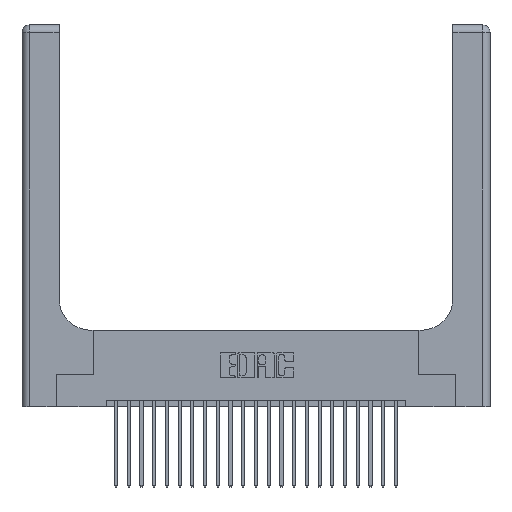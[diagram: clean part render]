
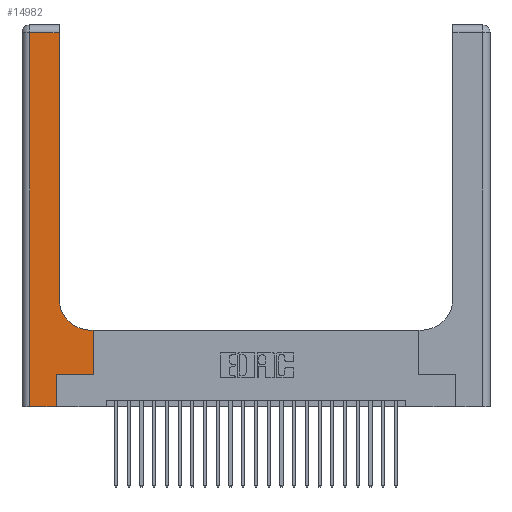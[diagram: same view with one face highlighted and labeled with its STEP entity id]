
A CAD part, top view. The second image highlights one B-rep face of the part: STEP entity #14982.
In plain terms, the highlighted planar face has unit normal (0, 0, 1).
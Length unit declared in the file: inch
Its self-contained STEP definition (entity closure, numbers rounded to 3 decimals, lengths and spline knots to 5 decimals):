
#500 = VERTEX_POINT ( 'NONE', #14511 ) ;
#1380 = AXIS2_PLACEMENT_3D ( 'NONE', #7023, #3087, #8470 ) ;
#1766 = EDGE_CURVE ( 'NONE', #5076, #25313, #13003, .T. ) ;
#1852 = DIRECTION ( 'NONE',  ( 0., 0., -1. ) ) ;
#2378 = LINE ( 'NONE', #7944, #5804 ) ;
#2521 = EDGE_CURVE ( 'NONE', #20014, #14028, #17039, .T. ) ;
#2746 = DIRECTION ( 'NONE',  ( 1., 0., 0. ) ) ;
#3087 = DIRECTION ( 'NONE',  ( 0., 0., -1. ) ) ;
#3136 = CARTESIAN_POINT ( 'NONE',  ( 0., 2.94, 0.37 ) ) ;
#3296 = VERTEX_POINT ( 'NONE', #9178 ) ;
#3462 = EDGE_CURVE ( 'NONE', #7526, #5076, #9514, .T. ) ;
#3810 = VECTOR ( 'NONE', #18272, 39.37008 ) ;
#4483 = EDGE_CURVE ( 'NONE', #500, #9376, #19374, .T. ) ;
#4712 = ORIENTED_EDGE ( 'NONE', *, *, #5299, .T. ) ;
#4729 = VECTOR ( 'NONE', #17124, 39.37008 ) ;
#4816 = PLANE ( 'NONE',  #1380 ) ;
#5076 = VERTEX_POINT ( 'NONE', #23643 ) ;
#5299 = EDGE_CURVE ( 'NONE', #21081, #20014, #17511, .T. ) ;
#5738 = ORIENTED_EDGE ( 'NONE', *, *, #4483, .T. ) ;
#5804 = VECTOR ( 'NONE', #7861, 39.37008 ) ;
#5982 = EDGE_CURVE ( 'NONE', #25313, #500, #2378, .T. ) ;
#6033 = CARTESIAN_POINT ( 'NONE',  ( 0.06, 0., 0.37 ) ) ;
#6135 = CARTESIAN_POINT ( 'NONE',  ( 0.06, 3., 0.37 ) ) ;
#6391 = VECTOR ( 'NONE', #8173, 39.37008 ) ;
#7023 = CARTESIAN_POINT ( 'NONE',  ( 0., 3., 0.37 ) ) ;
#7526 = VERTEX_POINT ( 'NONE', #17850 ) ;
#7823 = DIRECTION ( 'NONE',  ( 0., 1., 0. ) ) ;
#7861 = DIRECTION ( 'NONE',  ( 0., 1., 0. ) ) ;
#7944 = CARTESIAN_POINT ( 'NONE',  ( 0.5585, 0.25, 0.37 ) ) ;
#8173 = DIRECTION ( 'NONE',  ( 1., 0., 0. ) ) ;
#8470 = DIRECTION ( 'NONE',  ( -1., 0., 0. ) ) ;
#8827 = LINE ( 'NONE', #22658, #4729 ) ;
#9028 = EDGE_CURVE ( 'NONE', #3296, #21081, #8827, .T. ) ;
#9073 = CIRCLE ( 'NONE', #20155, 0.25 ) ;
#9178 = CARTESIAN_POINT ( 'NONE',  ( 0.2915, 0.85, 0.37 ) ) ;
#9376 = VERTEX_POINT ( 'NONE', #17472 ) ;
#9514 = LINE ( 'NONE', #13137, #20052 ) ;
#10505 = CARTESIAN_POINT ( 'NONE',  ( 0.2915, 2.94, 0.37 ) ) ;
#11107 = CARTESIAN_POINT ( 'NONE',  ( 0.5585, 0.25, 0.37 ) ) ;
#12345 = CARTESIAN_POINT ( 'NONE',  ( 0.2915, 0.6, 0.37 ) ) ;
#12406 = ORIENTED_EDGE ( 'NONE', *, *, #9028, .T. ) ;
#12634 = VECTOR ( 'NONE', #17827, 39.37008 ) ;
#13003 = LINE ( 'NONE', #20391, #13927 ) ;
#13137 = CARTESIAN_POINT ( 'NONE',  ( 0.269, 0., 0.37 ) ) ;
#13927 = VECTOR ( 'NONE', #2746, 39.37008 ) ;
#14028 = VERTEX_POINT ( 'NONE', #6033 ) ;
#14294 = FACE_OUTER_BOUND ( 'NONE', #24519, .T. ) ;
#14511 = CARTESIAN_POINT ( 'NONE',  ( 0.5585, 0.6, 0.37 ) ) ;
#14982 = ADVANCED_FACE ( 'NONE', ( #14294 ), #4816, .F. ) ;
#15937 = CARTESIAN_POINT ( 'NONE',  ( 0., 0., 0.37 ) ) ;
#16736 = ORIENTED_EDGE ( 'NONE', *, *, #1766, .T. ) ;
#17039 = LINE ( 'NONE', #6135, #12634 ) ;
#17124 = DIRECTION ( 'NONE',  ( 0., 1., 0. ) ) ;
#17213 = ORIENTED_EDGE ( 'NONE', *, *, #3462, .T. ) ;
#17472 = CARTESIAN_POINT ( 'NONE',  ( 0.5415, 0.6, 0.37 ) ) ;
#17511 = LINE ( 'NONE', #3136, #18398 ) ;
#17641 = LINE ( 'NONE', #15937, #6391 ) ;
#17827 = DIRECTION ( 'NONE',  ( 0., -1., 0. ) ) ;
#17850 = CARTESIAN_POINT ( 'NONE',  ( 0.269, 0., 0.37 ) ) ;
#18187 = EDGE_CURVE ( 'NONE', #14028, #7526, #17641, .T. ) ;
#18272 = DIRECTION ( 'NONE',  ( -1., 0., 0. ) ) ;
#18398 = VECTOR ( 'NONE', #19476, 39.37008 ) ;
#19374 = LINE ( 'NONE', #12345, #3810 ) ;
#19476 = DIRECTION ( 'NONE',  ( -1., 0., 0. ) ) ;
#20014 = VERTEX_POINT ( 'NONE', #22826 ) ;
#20052 = VECTOR ( 'NONE', #7823, 39.37008 ) ;
#20155 = AXIS2_PLACEMENT_3D ( 'NONE', #21852, #1852, #23727 ) ;
#20391 = CARTESIAN_POINT ( 'NONE',  ( 0.269, 0.25, 0.37 ) ) ;
#21081 = VERTEX_POINT ( 'NONE', #10505 ) ;
#21398 = ORIENTED_EDGE ( 'NONE', *, *, #5982, .T. ) ;
#21852 = CARTESIAN_POINT ( 'NONE',  ( 0.5415, 0.85, 0.37 ) ) ;
#22658 = CARTESIAN_POINT ( 'NONE',  ( 0.2915, 3., 0.37 ) ) ;
#22693 = EDGE_CURVE ( 'NONE', #9376, #3296, #9073, .T. ) ;
#22826 = CARTESIAN_POINT ( 'NONE',  ( 0.06, 2.94, 0.37 ) ) ;
#23643 = CARTESIAN_POINT ( 'NONE',  ( 0.269, 0.25, 0.37 ) ) ;
#23727 = DIRECTION ( 'NONE',  ( 1., 0., 0. ) ) ;
#23877 = ORIENTED_EDGE ( 'NONE', *, *, #18187, .T. ) ;
#24519 = EDGE_LOOP ( 'NONE', ( #12406, #4712, #24680, #23877, #17213, #16736, #21398, #5738, #25406 ) ) ;
#24680 = ORIENTED_EDGE ( 'NONE', *, *, #2521, .T. ) ;
#25313 = VERTEX_POINT ( 'NONE', #11107 ) ;
#25406 = ORIENTED_EDGE ( 'NONE', *, *, #22693, .T. ) ;
